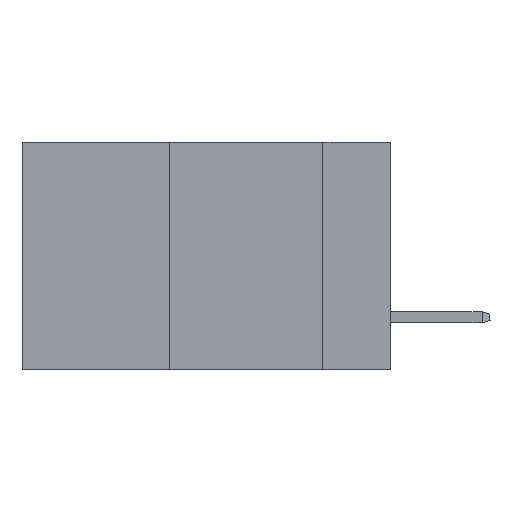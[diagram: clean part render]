
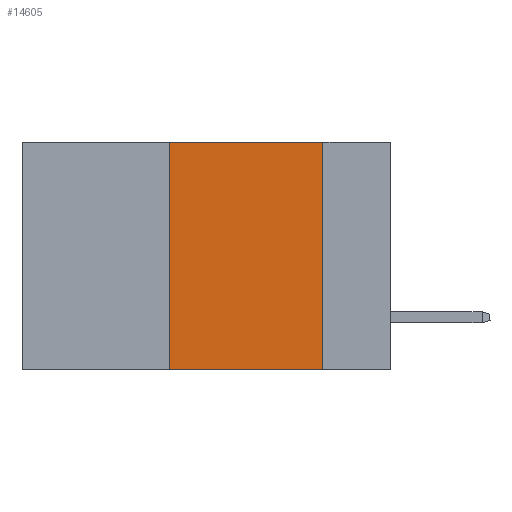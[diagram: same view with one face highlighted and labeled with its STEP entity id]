
A CAD part, left-side view. The second image highlights one B-rep face of the part: STEP entity #14605.
In plain terms, the highlighted planar face has unit normal (-1, 0, 0).
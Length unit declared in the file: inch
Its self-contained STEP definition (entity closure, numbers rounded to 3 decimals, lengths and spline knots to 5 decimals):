
#542 = DIRECTION ( 'NONE',  ( 0., -1., 0. ) ) ;
#1259 = DIRECTION ( 'NONE',  ( 0., 0., -1. ) ) ;
#1351 = CARTESIAN_POINT ( 'NONE',  ( 0., 0.36, 0. ) ) ;
#1600 = PLANE ( 'NONE',  #2911 ) ;
#2653 = VECTOR ( 'NONE', #1259, 39.37008 ) ;
#2872 = DIRECTION ( 'NONE',  ( 0., 0., -1. ) ) ;
#2893 = LINE ( 'NONE', #1351, #4665 ) ;
#2911 = AXIS2_PLACEMENT_3D ( 'NONE', #3984, #9179, #2872 ) ;
#3638 = DIRECTION ( 'NONE',  ( 0., -1., 0. ) ) ;
#3984 = CARTESIAN_POINT ( 'NONE',  ( 0., 0.6, 0. ) ) ;
#4460 = CARTESIAN_POINT ( 'NONE',  ( 0., 0.11, 0. ) ) ;
#4665 = VECTOR ( 'NONE', #15212, 39.37008 ) ;
#5144 = ORIENTED_EDGE ( 'NONE', *, *, #14181, .T. ) ;
#5636 = EDGE_LOOP ( 'NONE', ( #10556, #6769, #12782, #5144 ) ) ;
#6769 = ORIENTED_EDGE ( 'NONE', *, *, #7958, .F. ) ;
#7354 = VERTEX_POINT ( 'NONE', #13652 ) ;
#7452 = EDGE_CURVE ( 'NONE', #7936, #7354, #2893, .T. ) ;
#7936 = VERTEX_POINT ( 'NONE', #13742 ) ;
#7958 = EDGE_CURVE ( 'NONE', #7354, #13439, #16193, .T. ) ;
#8006 = VERTEX_POINT ( 'NONE', #10505 ) ;
#8893 = LINE ( 'NONE', #12213, #15244 ) ;
#9018 = CARTESIAN_POINT ( 'NONE',  ( 0., 0.6, 0. ) ) ;
#9179 = DIRECTION ( 'NONE',  ( 1., 0., 0. ) ) ;
#9675 = EDGE_CURVE ( 'NONE', #13439, #8006, #15291, .T. ) ;
#10505 = CARTESIAN_POINT ( 'NONE',  ( 0., 0.11, -0.37 ) ) ;
#10556 = ORIENTED_EDGE ( 'NONE', *, *, #9675, .F. ) ;
#11502 = CARTESIAN_POINT ( 'NONE',  ( 0., 0.11, 0. ) ) ;
#12213 = CARTESIAN_POINT ( 'NONE',  ( 0., 0.6, -0.37 ) ) ;
#12782 = ORIENTED_EDGE ( 'NONE', *, *, #7452, .F. ) ;
#13439 = VERTEX_POINT ( 'NONE', #4460 ) ;
#13652 = CARTESIAN_POINT ( 'NONE',  ( 0., 0.36, 0. ) ) ;
#13742 = CARTESIAN_POINT ( 'NONE',  ( 0., 0.36, -0.37 ) ) ;
#14181 = EDGE_CURVE ( 'NONE', #7936, #8006, #8893, .T. ) ;
#14605 = ADVANCED_FACE ( 'NONE', ( #15241 ), #1600, .F. ) ;
#14782 = VECTOR ( 'NONE', #542, 39.37008 ) ;
#15212 = DIRECTION ( 'NONE',  ( 0., 0., 1. ) ) ;
#15241 = FACE_OUTER_BOUND ( 'NONE', #5636, .T. ) ;
#15244 = VECTOR ( 'NONE', #3638, 39.37008 ) ;
#15291 = LINE ( 'NONE', #11502, #2653 ) ;
#16193 = LINE ( 'NONE', #9018, #14782 ) ;
